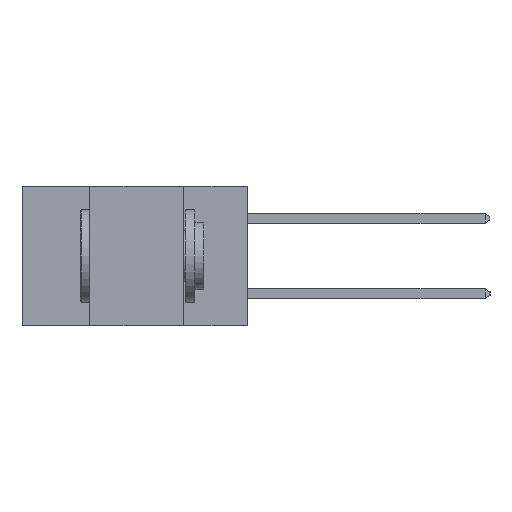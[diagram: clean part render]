
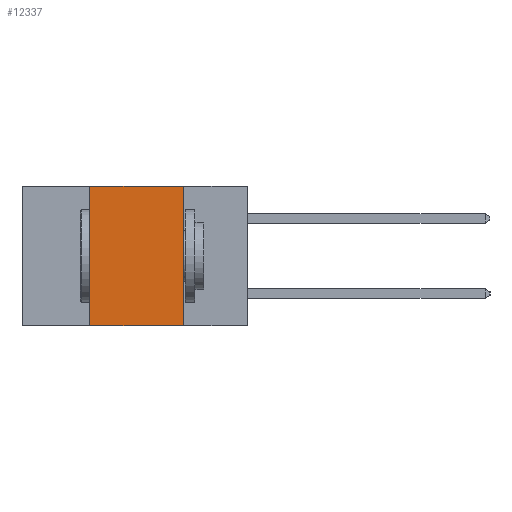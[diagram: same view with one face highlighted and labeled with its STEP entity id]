
A CAD part, left-side view. The second image highlights one B-rep face of the part: STEP entity #12337.
In plain terms, the highlighted planar face has unit normal (-1, 0, 0).
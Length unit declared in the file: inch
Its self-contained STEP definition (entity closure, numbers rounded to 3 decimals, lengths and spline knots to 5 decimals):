
#502 = ORIENTED_EDGE ( 'NONE', *, *, #3654, .F. ) ;
#652 = EDGE_CURVE ( 'NONE', #11752, #1073, #14177, .T. ) ;
#1073 = VERTEX_POINT ( 'NONE', #16199 ) ;
#1208 = VERTEX_POINT ( 'NONE', #11516 ) ;
#1658 = EDGE_CURVE ( 'NONE', #11752, #18408, #10245, .T. ) ;
#1801 = VECTOR ( 'NONE', #14712, 39.37008 ) ;
#2650 = EDGE_CURVE ( 'NONE', #18408, #1208, #8361, .T. ) ;
#2925 = CARTESIAN_POINT ( 'NONE',  ( 0., 0.42, 0. ) ) ;
#2935 = DIRECTION ( 'NONE',  ( 0., -1., 0. ) ) ;
#3559 = ORIENTED_EDGE ( 'NONE', *, *, #652, .T. ) ;
#3654 = EDGE_CURVE ( 'NONE', #1208, #1073, #7394, .T. ) ;
#4021 = ORIENTED_EDGE ( 'NONE', *, *, #2650, .F. ) ;
#4094 = CARTESIAN_POINT ( 'NONE',  ( 0., 0.42, -0.37 ) ) ;
#4592 = DIRECTION ( 'NONE',  ( 1., 0., 0. ) ) ;
#7234 = CARTESIAN_POINT ( 'NONE',  ( 0., 0.6, -0.37 ) ) ;
#7394 = LINE ( 'NONE', #16832, #14745 ) ;
#7609 = PLANE ( 'NONE',  #14507 ) ;
#8361 = LINE ( 'NONE', #9661, #16132 ) ;
#9661 = CARTESIAN_POINT ( 'NONE',  ( 0., 0.6, 0. ) ) ;
#9830 = DIRECTION ( 'NONE',  ( 0., -1., 0. ) ) ;
#10245 = LINE ( 'NONE', #18970, #1801 ) ;
#11516 = CARTESIAN_POINT ( 'NONE',  ( 0., 0.17, 0. ) ) ;
#11529 = ORIENTED_EDGE ( 'NONE', *, *, #1658, .F. ) ;
#11752 = VERTEX_POINT ( 'NONE', #4094 ) ;
#12337 = ADVANCED_FACE ( 'NONE', ( #15861 ), #7609, .F. ) ;
#13568 = CARTESIAN_POINT ( 'NONE',  ( 0., 0.6, 0. ) ) ;
#14177 = LINE ( 'NONE', #7234, #17545 ) ;
#14507 = AXIS2_PLACEMENT_3D ( 'NONE', #13568, #4592, #14991 ) ;
#14712 = DIRECTION ( 'NONE',  ( 0., 0., 1. ) ) ;
#14745 = VECTOR ( 'NONE', #16647, 39.37008 ) ;
#14991 = DIRECTION ( 'NONE',  ( 0., 0., -1. ) ) ;
#15861 = FACE_OUTER_BOUND ( 'NONE', #18785, .T. ) ;
#16132 = VECTOR ( 'NONE', #9830, 39.37008 ) ;
#16199 = CARTESIAN_POINT ( 'NONE',  ( 0., 0.17, -0.37 ) ) ;
#16647 = DIRECTION ( 'NONE',  ( 0., 0., -1. ) ) ;
#16832 = CARTESIAN_POINT ( 'NONE',  ( 0., 0.17, -0.37 ) ) ;
#17545 = VECTOR ( 'NONE', #2935, 39.37008 ) ;
#18408 = VERTEX_POINT ( 'NONE', #2925 ) ;
#18785 = EDGE_LOOP ( 'NONE', ( #502, #4021, #11529, #3559 ) ) ;
#18970 = CARTESIAN_POINT ( 'NONE',  ( 0., 0.42, -0.37 ) ) ;
